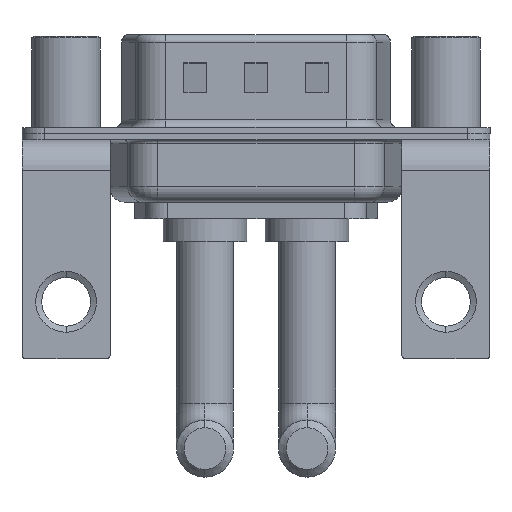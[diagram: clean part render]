
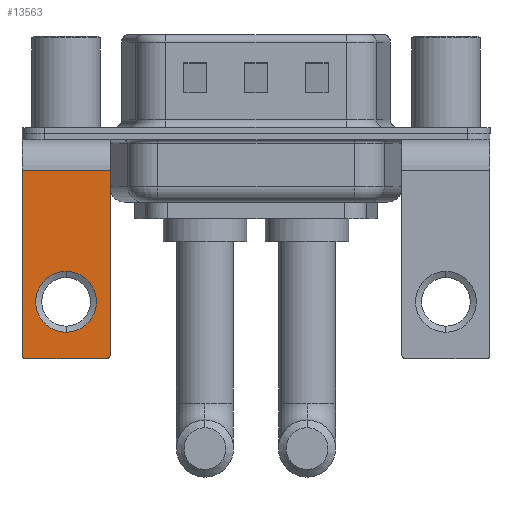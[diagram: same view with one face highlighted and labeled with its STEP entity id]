
A CAD part, front view. The second image highlights one B-rep face of the part: STEP entity #13563.
In plain terms, the highlighted planar face has unit normal (0, -1, 0).
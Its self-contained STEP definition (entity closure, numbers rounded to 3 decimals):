
#293 = CARTESIAN_POINT ( 'NONE',  ( 0., -6.25, -11.07 ) ) ;
#338 = ORIENTED_EDGE ( 'NONE', *, *, #15807, .T. ) ;
#722 = VERTEX_POINT ( 'NONE', #12234 ) ;
#983 = CARTESIAN_POINT ( 'NONE',  ( -2.9, -6.25, -14.55 ) ) ;
#1109 = CIRCLE ( 'NONE', #5754, 0.25 ) ;
#1276 = CIRCLE ( 'NONE', #3447, 2. ) ;
#1425 = ORIENTED_EDGE ( 'NONE', *, *, #3401, .T. ) ;
#1629 = EDGE_CURVE ( 'NONE', #9117, #2879, #14571, .T. ) ;
#1657 = DIRECTION ( 'NONE',  ( 0., 0., -1. ) ) ;
#1827 = EDGE_CURVE ( 'NONE', #722, #2879, #1109, .T. ) ;
#2146 = DIRECTION ( 'NONE',  ( 0., -1., 0. ) ) ;
#2370 = DIRECTION ( 'NONE',  ( 0., 1., 0. ) ) ;
#2660 = DIRECTION ( 'NONE',  ( -1., 0., 0. ) ) ;
#2844 = CARTESIAN_POINT ( 'NONE',  ( 2.9, -6.25, -2.4 ) ) ;
#2879 = VERTEX_POINT ( 'NONE', #14828 ) ;
#3023 = DIRECTION ( 'NONE',  ( 0., 0., 1. ) ) ;
#3240 = VERTEX_POINT ( 'NONE', #983 ) ;
#3401 = EDGE_CURVE ( 'NONE', #12332, #9640, #4370, .T. ) ;
#3447 = AXIS2_PLACEMENT_3D ( 'NONE', #6870, #14914, #13715 ) ;
#3555 = PLANE ( 'NONE',  #9133 ) ;
#3722 = CARTESIAN_POINT ( 'NONE',  ( 2.9, -6.25, -2.4 ) ) ;
#3930 = LINE ( 'NONE', #9427, #7969 ) ;
#4036 = EDGE_CURVE ( 'NONE', #9117, #5860, #7634, .T. ) ;
#4136 = EDGE_CURVE ( 'NONE', #722, #5014, #3930, .T. ) ;
#4217 = CARTESIAN_POINT ( 'NONE',  ( 0., -6.25, -13.07 ) ) ;
#4370 = CIRCLE ( 'NONE', #8766, 2. ) ;
#4420 = AXIS2_PLACEMENT_3D ( 'NONE', #10025, #2146, #3023 ) ;
#4666 = EDGE_CURVE ( 'NONE', #5860, #3240, #8825, .T. ) ;
#5009 = DIRECTION ( 'NONE',  ( 0., 0., 1. ) ) ;
#5014 = VERTEX_POINT ( 'NONE', #10118 ) ;
#5141 = DIRECTION ( 'NONE',  ( 0., 0., 1. ) ) ;
#5226 = VECTOR ( 'NONE', #11638, 1000. ) ;
#5311 = ORIENTED_EDGE ( 'NONE', *, *, #4666, .T. ) ;
#5411 = DIRECTION ( 'NONE',  ( 0., 1., 0. ) ) ;
#5754 = AXIS2_PLACEMENT_3D ( 'NONE', #11567, #16679, #5141 ) ;
#5860 = VERTEX_POINT ( 'NONE', #13173 ) ;
#5958 = ORIENTED_EDGE ( 'NONE', *, *, #4036, .T. ) ;
#6066 = CIRCLE ( 'NONE', #4420, 0.25 ) ;
#6777 = CARTESIAN_POINT ( 'NONE',  ( 0., -6.25, -9.07 ) ) ;
#6870 = CARTESIAN_POINT ( 'NONE',  ( 0., -6.25, -11.07 ) ) ;
#7634 = LINE ( 'NONE', #12850, #9856 ) ;
#7673 = FACE_BOUND ( 'NONE', #15551, .T. ) ;
#7906 = EDGE_CURVE ( 'NONE', #3240, #5014, #6066, .T. ) ;
#7969 = VECTOR ( 'NONE', #2660, 1000. ) ;
#8448 = VECTOR ( 'NONE', #1657, 1000. ) ;
#8626 = EDGE_LOOP ( 'NONE', ( #5311, #9743, #11186, #10230, #10687, #5958 ) ) ;
#8766 = AXIS2_PLACEMENT_3D ( 'NONE', #293, #5411, #15839 ) ;
#8825 = LINE ( 'NONE', #15647, #5226 ) ;
#9117 = VERTEX_POINT ( 'NONE', #15198 ) ;
#9133 = AXIS2_PLACEMENT_3D ( 'NONE', #3722, #2370, #5009 ) ;
#9427 = CARTESIAN_POINT ( 'NONE',  ( 2.9, -6.25, -14.8 ) ) ;
#9640 = VERTEX_POINT ( 'NONE', #6777 ) ;
#9743 = ORIENTED_EDGE ( 'NONE', *, *, #7906, .T. ) ;
#9856 = VECTOR ( 'NONE', #15501, 1000. ) ;
#10025 = CARTESIAN_POINT ( 'NONE',  ( -2.65, -6.25, -14.55 ) ) ;
#10118 = CARTESIAN_POINT ( 'NONE',  ( -2.65, -6.25, -14.8 ) ) ;
#10230 = ORIENTED_EDGE ( 'NONE', *, *, #1827, .T. ) ;
#10687 = ORIENTED_EDGE ( 'NONE', *, *, #1629, .F. ) ;
#11186 = ORIENTED_EDGE ( 'NONE', *, *, #4136, .F. ) ;
#11567 = CARTESIAN_POINT ( 'NONE',  ( 2.65, -6.25, -14.55 ) ) ;
#11638 = DIRECTION ( 'NONE',  ( 0., 0., -1. ) ) ;
#12234 = CARTESIAN_POINT ( 'NONE',  ( 2.65, -6.25, -14.8 ) ) ;
#12332 = VERTEX_POINT ( 'NONE', #4217 ) ;
#12850 = CARTESIAN_POINT ( 'NONE',  ( 2.9, -6.25, -2.4 ) ) ;
#13173 = CARTESIAN_POINT ( 'NONE',  ( -2.9, -6.25, -2.4 ) ) ;
#13563 = ADVANCED_FACE ( 'NONE', ( #7673, #15113 ), #3555, .F. ) ;
#13715 = DIRECTION ( 'NONE',  ( 0., 0., 1. ) ) ;
#14571 = LINE ( 'NONE', #2844, #8448 ) ;
#14828 = CARTESIAN_POINT ( 'NONE',  ( 2.9, -6.25, -14.55 ) ) ;
#14914 = DIRECTION ( 'NONE',  ( 0., 1., 0. ) ) ;
#15113 = FACE_OUTER_BOUND ( 'NONE', #8626, .T. ) ;
#15198 = CARTESIAN_POINT ( 'NONE',  ( 2.9, -6.25, -2.4 ) ) ;
#15501 = DIRECTION ( 'NONE',  ( -1., 0., 0. ) ) ;
#15551 = EDGE_LOOP ( 'NONE', ( #1425, #338 ) ) ;
#15647 = CARTESIAN_POINT ( 'NONE',  ( -2.9, -6.25, -2.4 ) ) ;
#15807 = EDGE_CURVE ( 'NONE', #9640, #12332, #1276, .T. ) ;
#15839 = DIRECTION ( 'NONE',  ( 0., 0., 1. ) ) ;
#16679 = DIRECTION ( 'NONE',  ( 0., -1., 0. ) ) ;
